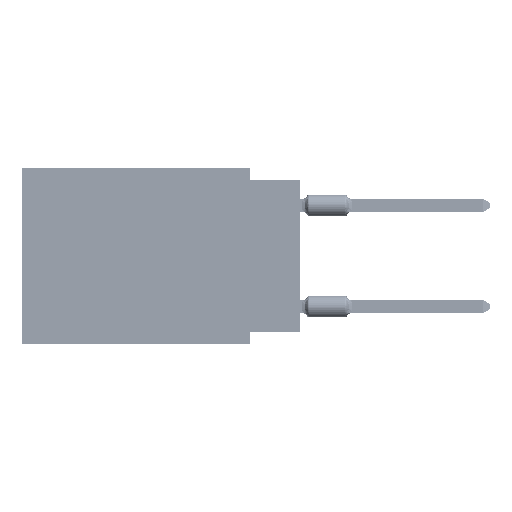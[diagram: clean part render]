
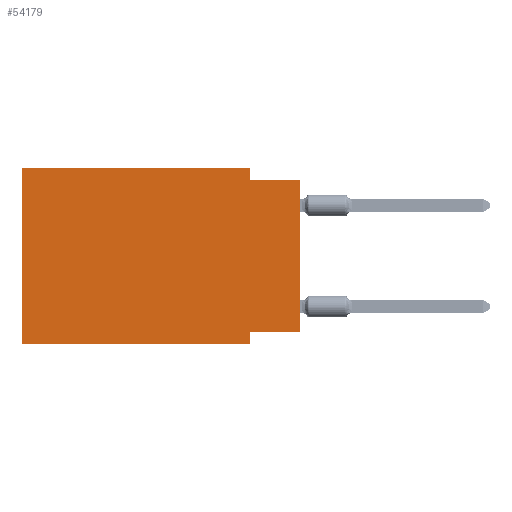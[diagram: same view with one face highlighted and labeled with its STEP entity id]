
A CAD part, left-side view. The second image highlights one B-rep face of the part: STEP entity #54179.
In plain terms, the highlighted planar face has unit normal (-1, 0, 0).
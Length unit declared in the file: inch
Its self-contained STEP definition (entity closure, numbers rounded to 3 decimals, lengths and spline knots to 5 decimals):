
#958 = PLANE ( 'NONE',  #18088 ) ;
#1430 = DIRECTION ( 'NONE',  ( 0., 0., -1. ) ) ;
#2085 = VERTEX_POINT ( 'NONE', #41368 ) ;
#3122 = LINE ( 'NONE', #72832, #73369 ) ;
#5671 = VERTEX_POINT ( 'NONE', #73724 ) ;
#5957 = DIRECTION ( 'NONE',  ( 1., 0., 0. ) ) ;
#6442 = EDGE_CURVE ( 'NONE', #5671, #47799, #15276, .T. ) ;
#6601 = LINE ( 'NONE', #41628, #7687 ) ;
#7687 = VECTOR ( 'NONE', #53423, 39.37008 ) ;
#8456 = DIRECTION ( 'NONE',  ( 0., 1., 0. ) ) ;
#9140 = CARTESIAN_POINT ( 'NONE',  ( 0., 0.55, 0. ) ) ;
#9258 = CARTESIAN_POINT ( 'NONE',  ( 0., 0.55, -0.35 ) ) ;
#11938 = VERTEX_POINT ( 'NONE', #9258 ) ;
#13529 = LINE ( 'NONE', #71431, #52754 ) ;
#14083 = VERTEX_POINT ( 'NONE', #47517 ) ;
#15276 = LINE ( 'NONE', #62485, #57292 ) ;
#15811 = VERTEX_POINT ( 'NONE', #34920 ) ;
#16874 = DIRECTION ( 'NONE',  ( 0., 0., 1. ) ) ;
#18088 = AXIS2_PLACEMENT_3D ( 'NONE', #29590, #5957, #35653 ) ;
#18594 = LINE ( 'NONE', #59726, #26569 ) ;
#18684 = ORIENTED_EDGE ( 'NONE', *, *, #21947, .F. ) ;
#19237 = DIRECTION ( 'NONE',  ( 0., -1., 0. ) ) ;
#21332 = LINE ( 'NONE', #9140, #38084 ) ;
#21780 = LINE ( 'NONE', #57950, #54034 ) ;
#21947 = EDGE_CURVE ( 'NONE', #2085, #36357, #18594, .T. ) ;
#22967 = LINE ( 'NONE', #56859, #36446 ) ;
#26569 = VECTOR ( 'NONE', #1430, 39.37008 ) ;
#27392 = EDGE_CURVE ( 'NONE', #14083, #5671, #13529, .T. ) ;
#27476 = CARTESIAN_POINT ( 'NONE',  ( 0., 0., -0.025 ) ) ;
#27890 = DIRECTION ( 'NONE',  ( 0., -1., 0. ) ) ;
#29590 = CARTESIAN_POINT ( 'NONE',  ( 0., 0.55, 0. ) ) ;
#32040 = DIRECTION ( 'NONE',  ( 0., 0., -1. ) ) ;
#32371 = EDGE_LOOP ( 'NONE', ( #63978, #65635, #64291, #65512, #74692, #50693, #18684, #59172 ) ) ;
#34920 = CARTESIAN_POINT ( 'NONE',  ( 0., 0., -0.325 ) ) ;
#35653 = DIRECTION ( 'NONE',  ( 0., 0., -1. ) ) ;
#36029 = EDGE_CURVE ( 'NONE', #15811, #42275, #22967, .T. ) ;
#36357 = VERTEX_POINT ( 'NONE', #49185 ) ;
#36446 = VECTOR ( 'NONE', #16874, 39.37008 ) ;
#38084 = VECTOR ( 'NONE', #38478, 39.37008 ) ;
#38478 = DIRECTION ( 'NONE',  ( 0., 0., 1. ) ) ;
#41368 = CARTESIAN_POINT ( 'NONE',  ( 0., 0.1, -0.325 ) ) ;
#41628 = CARTESIAN_POINT ( 'NONE',  ( 0., 0.55, -0.35 ) ) ;
#42275 = VERTEX_POINT ( 'NONE', #27476 ) ;
#46233 = EDGE_CURVE ( 'NONE', #11938, #14083, #21332, .T. ) ;
#47517 = CARTESIAN_POINT ( 'NONE',  ( 0., 0.55, 0. ) ) ;
#47799 = VERTEX_POINT ( 'NONE', #48684 ) ;
#48684 = CARTESIAN_POINT ( 'NONE',  ( 0., 0.1, -0.025 ) ) ;
#49185 = CARTESIAN_POINT ( 'NONE',  ( 0., 0.1, -0.35 ) ) ;
#50693 = ORIENTED_EDGE ( 'NONE', *, *, #60768, .T. ) ;
#52754 = VECTOR ( 'NONE', #19237, 39.37008 ) ;
#53423 = DIRECTION ( 'NONE',  ( 0., -1., 0. ) ) ;
#54034 = VECTOR ( 'NONE', #27890, 39.37008 ) ;
#54179 = ADVANCED_FACE ( 'NONE', ( #57388 ), #958, .F. ) ;
#56859 = CARTESIAN_POINT ( 'NONE',  ( 0., 0., 0. ) ) ;
#57292 = VECTOR ( 'NONE', #32040, 39.37008 ) ;
#57388 = FACE_OUTER_BOUND ( 'NONE', #32371, .T. ) ;
#57950 = CARTESIAN_POINT ( 'NONE',  ( 0., 0., -0.025 ) ) ;
#59172 = ORIENTED_EDGE ( 'NONE', *, *, #60824, .F. ) ;
#59726 = CARTESIAN_POINT ( 'NONE',  ( 0., 0.1, -0.35 ) ) ;
#60768 = EDGE_CURVE ( 'NONE', #11938, #36357, #6601, .T. ) ;
#60824 = EDGE_CURVE ( 'NONE', #15811, #2085, #3122, .T. ) ;
#62485 = CARTESIAN_POINT ( 'NONE',  ( 0., 0.1, 0. ) ) ;
#63978 = ORIENTED_EDGE ( 'NONE', *, *, #36029, .T. ) ;
#64291 = ORIENTED_EDGE ( 'NONE', *, *, #6442, .F. ) ;
#65512 = ORIENTED_EDGE ( 'NONE', *, *, #27392, .F. ) ;
#65635 = ORIENTED_EDGE ( 'NONE', *, *, #66644, .F. ) ;
#66644 = EDGE_CURVE ( 'NONE', #47799, #42275, #21780, .T. ) ;
#71431 = CARTESIAN_POINT ( 'NONE',  ( 0., 0.55, 0. ) ) ;
#72832 = CARTESIAN_POINT ( 'NONE',  ( 0., 0., -0.325 ) ) ;
#73369 = VECTOR ( 'NONE', #8456, 39.37008 ) ;
#73724 = CARTESIAN_POINT ( 'NONE',  ( 0., 0.1, 0. ) ) ;
#74692 = ORIENTED_EDGE ( 'NONE', *, *, #46233, .F. ) ;
